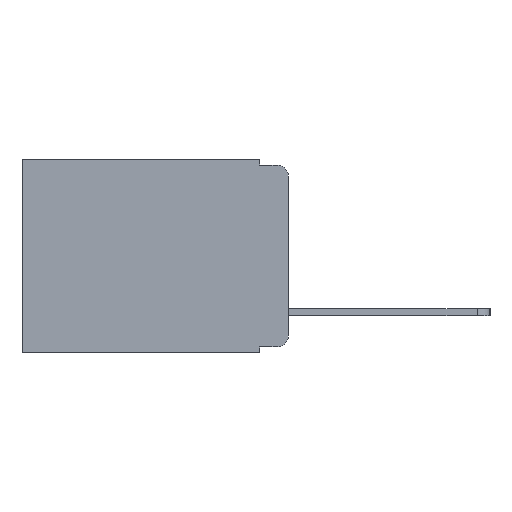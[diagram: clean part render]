
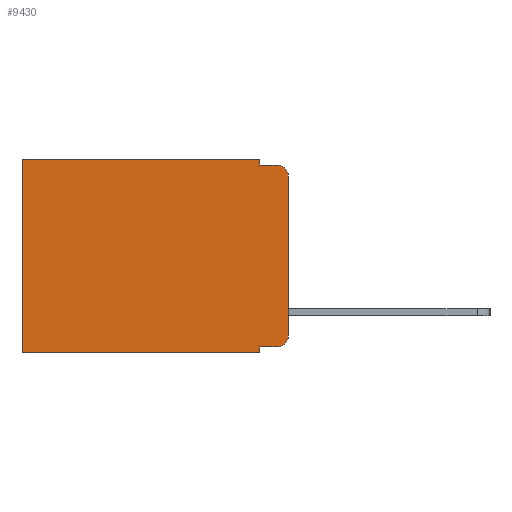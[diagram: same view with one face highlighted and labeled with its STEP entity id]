
A CAD part, left-side view. The second image highlights one B-rep face of the part: STEP entity #9430.
In plain terms, the highlighted planar face has unit normal (-1, 0, 0).
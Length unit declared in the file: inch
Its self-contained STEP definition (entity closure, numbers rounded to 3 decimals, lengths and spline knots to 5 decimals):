
#568 = CARTESIAN_POINT ( 'NONE',  ( 0.298, 0.051, -0.333 ) ) ;
#654 = AXIS2_PLACEMENT_3D ( 'NONE', #11671, #15012, #1677 ) ;
#816 = VERTEX_POINT ( 'NONE', #2249 ) ;
#869 = CARTESIAN_POINT ( 'NONE',  ( 0.298, 0., 0. ) ) ;
#924 = FACE_OUTER_BOUND ( 'NONE', #15623, .T. ) ;
#1147 = VERTEX_POINT ( 'NONE', #10625 ) ;
#1514 = PLANE ( 'NONE',  #9216 ) ;
#1618 = ORIENTED_EDGE ( 'NONE', *, *, #5464, .T. ) ;
#1677 = DIRECTION ( 'NONE',  ( 0., 0., -1. ) ) ;
#1797 = VECTOR ( 'NONE', #15583, 39.37008 ) ;
#2091 = DIRECTION ( 'NONE',  ( 0., 0., -1. ) ) ;
#2249 = CARTESIAN_POINT ( 'NONE',  ( 0.298, 0.473, -0.343 ) ) ;
#2647 = LINE ( 'NONE', #10292, #1797 ) ;
#2752 = ORIENTED_EDGE ( 'NONE', *, *, #10179, .T. ) ;
#2765 = CARTESIAN_POINT ( 'NONE',  ( 0.298, 0.051, -0.01 ) ) ;
#3049 = ORIENTED_EDGE ( 'NONE', *, *, #12619, .F. ) ;
#3149 = VECTOR ( 'NONE', #8439, 39.37008 ) ;
#3420 = VERTEX_POINT ( 'NONE', #5267 ) ;
#3551 = LINE ( 'NONE', #9609, #3149 ) ;
#3842 = LINE ( 'NONE', #568, #11910 ) ;
#4071 = DIRECTION ( 'NONE',  ( 0., -1., 0. ) ) ;
#4178 = CARTESIAN_POINT ( 'NONE',  ( 0.298, 0., 0. ) ) ;
#4443 = CARTESIAN_POINT ( 'NONE',  ( 0.298, 0.02, -0.03 ) ) ;
#4910 = CARTESIAN_POINT ( 'NONE',  ( 0.298, 0.051, -0.01 ) ) ;
#4925 = LINE ( 'NONE', #869, #9182 ) ;
#5021 = EDGE_CURVE ( 'NONE', #11597, #14960, #10814, .T. ) ;
#5224 = ORIENTED_EDGE ( 'NONE', *, *, #6801, .F. ) ;
#5267 = CARTESIAN_POINT ( 'NONE',  ( 0.298, 0.051, 0. ) ) ;
#5319 = ORIENTED_EDGE ( 'NONE', *, *, #13153, .F. ) ;
#5342 = ORIENTED_EDGE ( 'NONE', *, *, #7648, .T. ) ;
#5464 = EDGE_CURVE ( 'NONE', #3420, #7305, #2647, .T. ) ;
#5678 = DIRECTION ( 'NONE',  ( 0., 0., -1. ) ) ;
#5761 = LINE ( 'NONE', #15080, #8827 ) ;
#5852 = CARTESIAN_POINT ( 'NONE',  ( 0.298, 0.02, -0.01 ) ) ;
#5886 = EDGE_CURVE ( 'NONE', #10462, #11597, #3842, .T. ) ;
#6767 = DIRECTION ( 'NONE',  ( 1., 0., 0. ) ) ;
#6801 = EDGE_CURVE ( 'NONE', #10462, #1147, #5761, .T. ) ;
#7305 = VERTEX_POINT ( 'NONE', #13433 ) ;
#7648 = EDGE_CURVE ( 'NONE', #7305, #816, #15890, .T. ) ;
#7767 = ORIENTED_EDGE ( 'NONE', *, *, #9364, .F. ) ;
#7867 = LINE ( 'NONE', #11007, #11536 ) ;
#8244 = VECTOR ( 'NONE', #4071, 39.37008 ) ;
#8439 = DIRECTION ( 'NONE',  ( 0., 1., 0. ) ) ;
#8513 = EDGE_CURVE ( 'NONE', #3420, #15786, #7867, .T. ) ;
#8657 = LINE ( 'NONE', #2765, #8244 ) ;
#8827 = VECTOR ( 'NONE', #8964, 39.37008 ) ;
#8964 = DIRECTION ( 'NONE',  ( 0., 0., -1. ) ) ;
#9182 = VECTOR ( 'NONE', #14790, 39.37008 ) ;
#9216 = AXIS2_PLACEMENT_3D ( 'NONE', #4178, #6767, #15447 ) ;
#9225 = CIRCLE ( 'NONE', #13508, 0.02 ) ;
#9364 = EDGE_CURVE ( 'NONE', #15786, #13648, #8657, .T. ) ;
#9430 = ADVANCED_FACE ( 'NONE', ( #924 ), #1514, .F. ) ;
#9508 = CARTESIAN_POINT ( 'NONE',  ( 0.298, 0.02, -0.333 ) ) ;
#9609 = CARTESIAN_POINT ( 'NONE',  ( 0.298, 0., -0.343 ) ) ;
#10002 = ORIENTED_EDGE ( 'NONE', *, *, #8513, .F. ) ;
#10165 = ORIENTED_EDGE ( 'NONE', *, *, #5021, .T. ) ;
#10179 = EDGE_CURVE ( 'NONE', #13531, #13648, #9225, .T. ) ;
#10292 = CARTESIAN_POINT ( 'NONE',  ( 0.298, 0., 0. ) ) ;
#10462 = VERTEX_POINT ( 'NONE', #11168 ) ;
#10625 = CARTESIAN_POINT ( 'NONE',  ( 0.298, 0.051, -0.343 ) ) ;
#10706 = CARTESIAN_POINT ( 'NONE',  ( 0.298, 0., -0.03 ) ) ;
#10814 = CIRCLE ( 'NONE', #654, 0.02 ) ;
#11007 = CARTESIAN_POINT ( 'NONE',  ( 0.298, 0.051, 0. ) ) ;
#11168 = CARTESIAN_POINT ( 'NONE',  ( 0.298, 0.051, -0.333 ) ) ;
#11536 = VECTOR ( 'NONE', #2091, 39.37008 ) ;
#11597 = VERTEX_POINT ( 'NONE', #9508 ) ;
#11671 = CARTESIAN_POINT ( 'NONE',  ( 0.298, 0.02, -0.313 ) ) ;
#11858 = ORIENTED_EDGE ( 'NONE', *, *, #5886, .T. ) ;
#11910 = VECTOR ( 'NONE', #12551, 39.37008 ) ;
#11918 = DIRECTION ( 'NONE',  ( 0., 0., -1. ) ) ;
#12230 = VECTOR ( 'NONE', #11918, 39.37008 ) ;
#12551 = DIRECTION ( 'NONE',  ( 0., -1., 0. ) ) ;
#12619 = EDGE_CURVE ( 'NONE', #13531, #14960, #4925, .T. ) ;
#13153 = EDGE_CURVE ( 'NONE', #1147, #816, #3551, .T. ) ;
#13175 = CARTESIAN_POINT ( 'NONE',  ( 0.298, 0.473, 0. ) ) ;
#13212 = DIRECTION ( 'NONE',  ( -1., 0., 0. ) ) ;
#13433 = CARTESIAN_POINT ( 'NONE',  ( 0.298, 0.473, 0. ) ) ;
#13508 = AXIS2_PLACEMENT_3D ( 'NONE', #4443, #13212, #5678 ) ;
#13531 = VERTEX_POINT ( 'NONE', #10706 ) ;
#13648 = VERTEX_POINT ( 'NONE', #5852 ) ;
#14603 = CARTESIAN_POINT ( 'NONE',  ( 0.298, 0., -0.313 ) ) ;
#14790 = DIRECTION ( 'NONE',  ( 0., 0., -1. ) ) ;
#14960 = VERTEX_POINT ( 'NONE', #14603 ) ;
#15012 = DIRECTION ( 'NONE',  ( -1., 0., 0. ) ) ;
#15080 = CARTESIAN_POINT ( 'NONE',  ( 0.298, 0.051, 0. ) ) ;
#15447 = DIRECTION ( 'NONE',  ( 0., 0., -1. ) ) ;
#15583 = DIRECTION ( 'NONE',  ( 0., 1., 0. ) ) ;
#15623 = EDGE_LOOP ( 'NONE', ( #3049, #2752, #7767, #10002, #1618, #5342, #5319, #5224, #11858, #10165 ) ) ;
#15786 = VERTEX_POINT ( 'NONE', #4910 ) ;
#15890 = LINE ( 'NONE', #13175, #12230 ) ;
